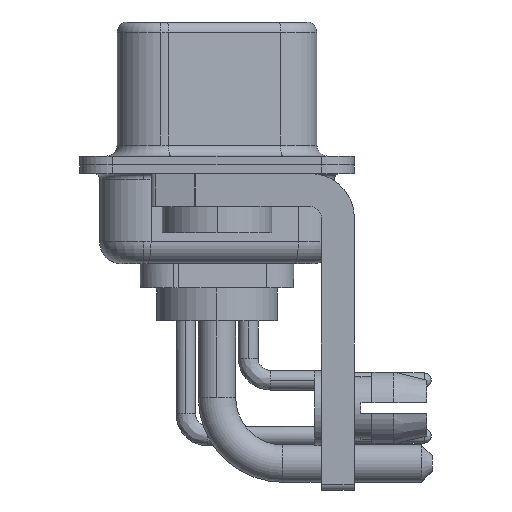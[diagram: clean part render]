
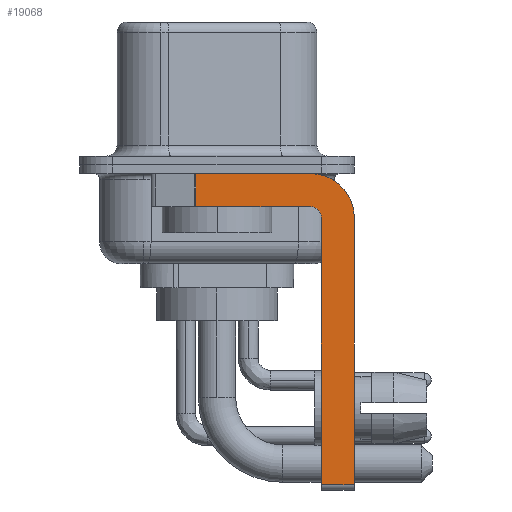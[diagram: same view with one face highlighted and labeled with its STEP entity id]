
A CAD part, left-side view. The second image highlights one B-rep face of the part: STEP entity #19068.
In plain terms, the highlighted planar face has unit normal (-1, 0, 0).
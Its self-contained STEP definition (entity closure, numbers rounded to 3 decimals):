
#395 = DIRECTION ( 'NONE',  ( 0., 0., 1. ) ) ;
#421 = VECTOR ( 'NONE', #13889, 1000. ) ;
#606 = CIRCLE ( 'NONE', #20894, 0.5 ) ;
#931 = EDGE_CURVE ( 'NONE', #10745, #17716, #3829, .T. ) ;
#1008 = LINE ( 'NONE', #9444, #5101 ) ;
#1102 = ORIENTED_EDGE ( 'NONE', *, *, #8807, .F. ) ;
#1730 = LINE ( 'NONE', #16521, #14747 ) ;
#2007 = DIRECTION ( 'NONE',  ( 0., -1., 0. ) ) ;
#2198 = DIRECTION ( 'NONE',  ( -1., 0., 0. ) ) ;
#2614 = CARTESIAN_POINT ( 'NONE',  ( -2.9, -4.25, -2.4 ) ) ;
#2949 = EDGE_CURVE ( 'NONE', #22671, #17716, #1008, .T. ) ;
#3123 = EDGE_CURVE ( 'NONE', #6398, #6632, #6748, .T. ) ;
#3829 = LINE ( 'NONE', #11992, #9394 ) ;
#4673 = ORIENTED_EDGE ( 'NONE', *, *, #3123, .F. ) ;
#5101 = VECTOR ( 'NONE', #17870, 1000. ) ;
#6398 = VERTEX_POINT ( 'NONE', #20204 ) ;
#6632 = VERTEX_POINT ( 'NONE', #17421 ) ;
#6748 = LINE ( 'NONE', #11040, #17890 ) ;
#7346 = CARTESIAN_POINT ( 'NONE',  ( -2.9, -4.25, -2.4 ) ) ;
#7475 = DIRECTION ( 'NONE',  ( 0., 0., -1. ) ) ;
#8603 = CIRCLE ( 'NONE', #19196, 2. ) ;
#8805 = VECTOR ( 'NONE', #12008, 1000. ) ;
#8807 = EDGE_CURVE ( 'NONE', #17401, #24285, #18296, .T. ) ;
#9394 = VECTOR ( 'NONE', #20668, 1000. ) ;
#9444 = CARTESIAN_POINT ( 'NONE',  ( -2.9, -4.25, -1.9 ) ) ;
#9579 = CARTESIAN_POINT ( 'NONE',  ( -2.9, -6.25, -14.55 ) ) ;
#10745 = VERTEX_POINT ( 'NONE', #20427 ) ;
#11040 = CARTESIAN_POINT ( 'NONE',  ( -2.9, -4.75, -14.8 ) ) ;
#11992 = CARTESIAN_POINT ( 'NONE',  ( -2.9, 0.978, -1.9 ) ) ;
#12008 = DIRECTION ( 'NONE',  ( 0., -1., 0. ) ) ;
#12069 = CARTESIAN_POINT ( 'NONE',  ( -2.9, 0.978, -1.9 ) ) ;
#12625 = DIRECTION ( 'NONE',  ( 0., 0., -1. ) ) ;
#12754 = CARTESIAN_POINT ( 'NONE',  ( -2.9, -4.25, -2.4 ) ) ;
#13298 = CARTESIAN_POINT ( 'NONE',  ( -2.9, -4.25, -1.9 ) ) ;
#13820 = LINE ( 'NONE', #22361, #8805 ) ;
#13889 = DIRECTION ( 'NONE',  ( 0., 0., -1. ) ) ;
#13981 = ORIENTED_EDGE ( 'NONE', *, *, #21862, .F. ) ;
#14747 = VECTOR ( 'NONE', #2007, 1000. ) ;
#14891 = EDGE_CURVE ( 'NONE', #6398, #24285, #13820, .T. ) ;
#15987 = ORIENTED_EDGE ( 'NONE', *, *, #22876, .F. ) ;
#16521 = CARTESIAN_POINT ( 'NONE',  ( -2.9, 3., -0.4 ) ) ;
#16738 = ORIENTED_EDGE ( 'NONE', *, *, #27190, .F. ) ;
#17059 = CARTESIAN_POINT ( 'NONE',  ( -2.9, -6.25, -2.4 ) ) ;
#17401 = VERTEX_POINT ( 'NONE', #17059 ) ;
#17421 = CARTESIAN_POINT ( 'NONE',  ( -2.9, -4.75, -2.4 ) ) ;
#17716 = VERTEX_POINT ( 'NONE', #12069 ) ;
#17870 = DIRECTION ( 'NONE',  ( 0., 1., 0. ) ) ;
#17890 = VECTOR ( 'NONE', #395, 1000. ) ;
#18296 = LINE ( 'NONE', #24636, #421 ) ;
#18693 = PLANE ( 'NONE',  #24816 ) ;
#18924 = ORIENTED_EDGE ( 'NONE', *, *, #14891, .T. ) ;
#18961 = DIRECTION ( 'NONE',  ( 1., 0., 0. ) ) ;
#19068 = ADVANCED_FACE ( 'NONE', ( #24899 ), #18693, .F. ) ;
#19196 = AXIS2_PLACEMENT_3D ( 'NONE', #7346, #26263, #7475 ) ;
#20204 = CARTESIAN_POINT ( 'NONE',  ( -2.9, -4.75, -14.55 ) ) ;
#20427 = CARTESIAN_POINT ( 'NONE',  ( -2.9, 0.978, -0.4 ) ) ;
#20668 = DIRECTION ( 'NONE',  ( 0., 0., -1. ) ) ;
#20894 = AXIS2_PLACEMENT_3D ( 'NONE', #2614, #2198, #21388 ) ;
#21369 = ORIENTED_EDGE ( 'NONE', *, *, #2949, .F. ) ;
#21388 = DIRECTION ( 'NONE',  ( 0., 0., 1. ) ) ;
#21862 = EDGE_CURVE ( 'NONE', #6632, #22671, #606, .T. ) ;
#22361 = CARTESIAN_POINT ( 'NONE',  ( -2.9, -4.25, -14.55 ) ) ;
#22671 = VERTEX_POINT ( 'NONE', #13298 ) ;
#22876 = EDGE_CURVE ( 'NONE', #27312, #17401, #8603, .T. ) ;
#23900 = CARTESIAN_POINT ( 'NONE',  ( -2.9, -4.25, -0.4 ) ) ;
#23957 = EDGE_LOOP ( 'NONE', ( #16738, #27184, #21369, #13981, #4673, #18924, #1102, #15987 ) ) ;
#24285 = VERTEX_POINT ( 'NONE', #9579 ) ;
#24636 = CARTESIAN_POINT ( 'NONE',  ( -2.9, -6.25, -2.4 ) ) ;
#24816 = AXIS2_PLACEMENT_3D ( 'NONE', #12754, #18961, #12625 ) ;
#24899 = FACE_OUTER_BOUND ( 'NONE', #23957, .T. ) ;
#26263 = DIRECTION ( 'NONE',  ( 1., 0., 0. ) ) ;
#27184 = ORIENTED_EDGE ( 'NONE', *, *, #931, .T. ) ;
#27190 = EDGE_CURVE ( 'NONE', #10745, #27312, #1730, .T. ) ;
#27312 = VERTEX_POINT ( 'NONE', #23900 ) ;
